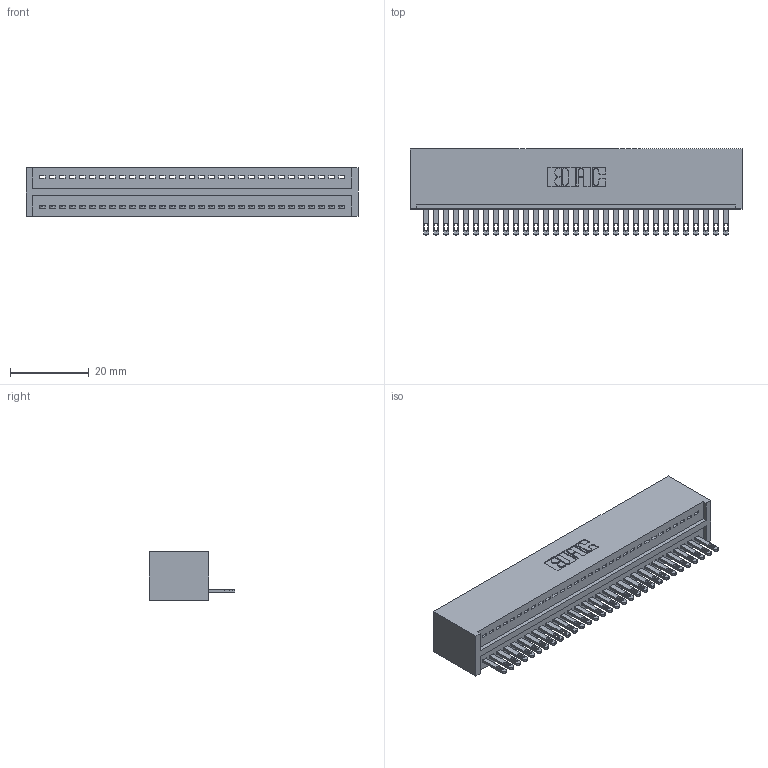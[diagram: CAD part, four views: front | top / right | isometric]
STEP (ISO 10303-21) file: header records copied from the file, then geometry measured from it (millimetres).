
FILE_DESCRIPTION (( 'STEP AP203' ), '1' );
FILE_NAME ('325-031-500-101.STEP', '2020-02-24T19:17:41', ( '' ), ( '' ), 'SwSTEP 2.0', 'SolidWorks 2016', '' );
FILE_SCHEMA (( 'CONFIG_CONTROL_DESIGN' ));
Length unit declared in the file: inch
Products named in the file (3): 325-031-500-101; 325-292-001_325-293-100; 325 Part_Lugless
Assembly tree (32 placements, depth 2):
  325-031-500-101
    325 Part_Lugless
    325-292-001_325-293-100  x31
Bounding box: 84.38 x 21.84 x 12.45 mm (x, y, z)
Volume: 11216.3 mm3; surface area: 12630.2 mm2
Topology: 32 solids, 32 shells, 1780 faces, 5495 edges, 3662 vertices
Faces by surface type: plane 1182, cylinder 598
Entity records: 20027 total; most frequent: CARTESIAN_POINT 3463, ORIENTED_EDGE 3430, DIRECTION 2937, EDGE_CURVE 1715, LINE 1591, VECTOR 1591, VERTEX_POINT 1142, AXIS2_PLACEMENT_3D 673
